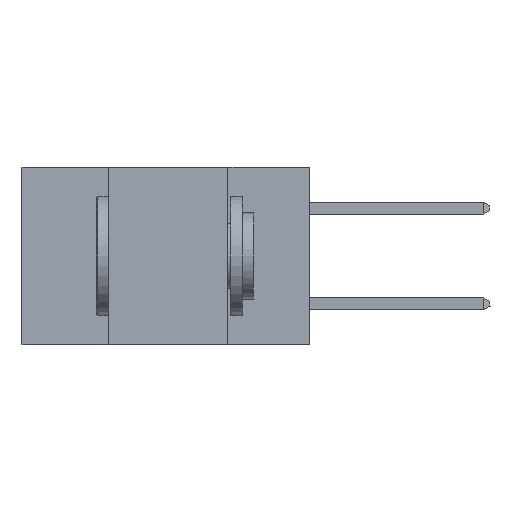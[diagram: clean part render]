
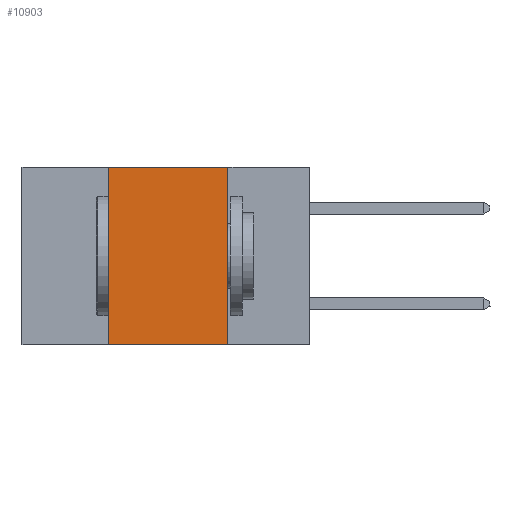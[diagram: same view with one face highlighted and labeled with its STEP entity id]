
A CAD part, left-side view. The second image highlights one B-rep face of the part: STEP entity #10903.
In plain terms, the highlighted planar face has unit normal (-1, 0, 0).
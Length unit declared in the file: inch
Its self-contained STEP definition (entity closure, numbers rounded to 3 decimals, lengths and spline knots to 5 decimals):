
#140 = ORIENTED_EDGE ( 'NONE', *, *, #20424, .T. ) ;
#246 = VERTEX_POINT ( 'NONE', #18923 ) ;
#1324 = VECTOR ( 'NONE', #19511, 39.37008 ) ;
#1953 = VERTEX_POINT ( 'NONE', #25546 ) ;
#2222 = AXIS2_PLACEMENT_3D ( 'NONE', #27501, #27692, #25626 ) ;
#2489 = CARTESIAN_POINT ( 'NONE',  ( 0., 0.6, -0.37 ) ) ;
#4134 = ORIENTED_EDGE ( 'NONE', *, *, #6677, .F. ) ;
#4463 = CARTESIAN_POINT ( 'NONE',  ( 0., 0.42, -0.37 ) ) ;
#5349 = LINE ( 'NONE', #2489, #14861 ) ;
#6422 = DIRECTION ( 'NONE',  ( 0., -1., 0. ) ) ;
#6424 = EDGE_CURVE ( 'NONE', #14054, #22770, #23982, .T. ) ;
#6677 = EDGE_CURVE ( 'NONE', #1953, #246, #27096, .T. ) ;
#10279 = DIRECTION ( 'NONE',  ( 0., 0., 1. ) ) ;
#10336 = ORIENTED_EDGE ( 'NONE', *, *, #6424, .F. ) ;
#10903 = ADVANCED_FACE ( 'NONE', ( #26602 ), #23375, .F. ) ;
#11816 = LINE ( 'NONE', #20076, #17827 ) ;
#14054 = VERTEX_POINT ( 'NONE', #4463 ) ;
#14861 = VECTOR ( 'NONE', #22437, 39.37008 ) ;
#16077 = EDGE_CURVE ( 'NONE', #22770, #1953, #11816, .T. ) ;
#17501 = EDGE_LOOP ( 'NONE', ( #4134, #20187, #10336, #140 ) ) ;
#17827 = VECTOR ( 'NONE', #6422, 39.37008 ) ;
#18599 = VECTOR ( 'NONE', #10279, 39.37008 ) ;
#18923 = CARTESIAN_POINT ( 'NONE',  ( 0., 0.17, -0.37 ) ) ;
#19511 = DIRECTION ( 'NONE',  ( 0., 0., -1. ) ) ;
#20076 = CARTESIAN_POINT ( 'NONE',  ( 0., 0.6, 0. ) ) ;
#20187 = ORIENTED_EDGE ( 'NONE', *, *, #16077, .F. ) ;
#20424 = EDGE_CURVE ( 'NONE', #14054, #246, #5349, .T. ) ;
#22437 = DIRECTION ( 'NONE',  ( 0., -1., 0. ) ) ;
#22770 = VERTEX_POINT ( 'NONE', #24940 ) ;
#23364 = CARTESIAN_POINT ( 'NONE',  ( 0., 0.42, 0. ) ) ;
#23375 = PLANE ( 'NONE',  #2222 ) ;
#23982 = LINE ( 'NONE', #23364, #18599 ) ;
#24138 = CARTESIAN_POINT ( 'NONE',  ( 0., 0.17, 0. ) ) ;
#24940 = CARTESIAN_POINT ( 'NONE',  ( 0., 0.42, 0. ) ) ;
#25546 = CARTESIAN_POINT ( 'NONE',  ( 0., 0.17, 0. ) ) ;
#25626 = DIRECTION ( 'NONE',  ( 0., 0., -1. ) ) ;
#26602 = FACE_OUTER_BOUND ( 'NONE', #17501, .T. ) ;
#27096 = LINE ( 'NONE', #24138, #1324 ) ;
#27501 = CARTESIAN_POINT ( 'NONE',  ( 0., 0.6, 0. ) ) ;
#27692 = DIRECTION ( 'NONE',  ( 1., 0., 0. ) ) ;
